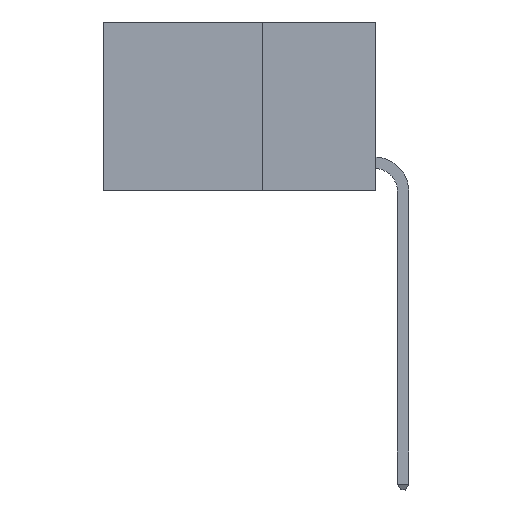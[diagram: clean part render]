
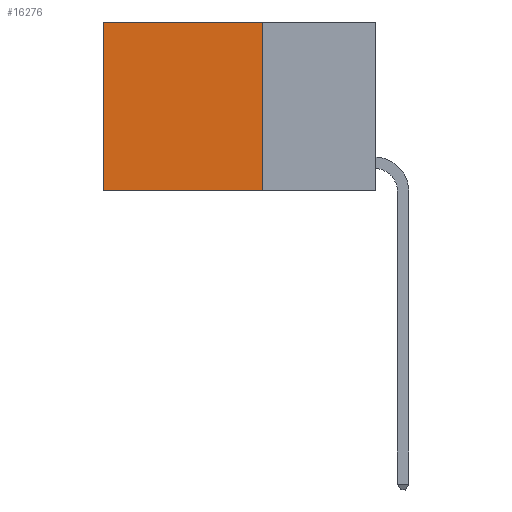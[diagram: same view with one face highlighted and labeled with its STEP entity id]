
A CAD part, left-side view. The second image highlights one B-rep face of the part: STEP entity #16276.
In plain terms, the highlighted planar face has unit normal (-1, 0, 0).
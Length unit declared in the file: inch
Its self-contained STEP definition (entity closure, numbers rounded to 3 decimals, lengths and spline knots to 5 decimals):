
#31 = CARTESIAN_POINT ( 'NONE',  ( 0.2625, 0.25, 0. ) ) ;
#176 = EDGE_CURVE ( 'NONE', #10624, #14972, #15602, .T. ) ;
#853 = LINE ( 'NONE', #31, #12790 ) ;
#1154 = CARTESIAN_POINT ( 'NONE',  ( 0.2625, 0.25, -0.37 ) ) ;
#1248 = DIRECTION ( 'NONE',  ( 0., 1., 0. ) ) ;
#1884 = DIRECTION ( 'NONE',  ( 0., 0., -1. ) ) ;
#3001 = VERTEX_POINT ( 'NONE', #10135 ) ;
#3259 = FACE_OUTER_BOUND ( 'NONE', #13086, .T. ) ;
#3706 = EDGE_CURVE ( 'NONE', #3001, #7408, #17821, .T. ) ;
#5511 = LINE ( 'NONE', #10163, #17362 ) ;
#6424 = CARTESIAN_POINT ( 'NONE',  ( 0.2625, 0.25, -0.37 ) ) ;
#7408 = VERTEX_POINT ( 'NONE', #14575 ) ;
#7544 = ORIENTED_EDGE ( 'NONE', *, *, #11592, .T. ) ;
#7986 = ORIENTED_EDGE ( 'NONE', *, *, #3706, .T. ) ;
#8156 = PLANE ( 'NONE',  #18578 ) ;
#9150 = VECTOR ( 'NONE', #14631, 39.37008 ) ;
#9650 = ORIENTED_EDGE ( 'NONE', *, *, #14235, .F. ) ;
#10135 = CARTESIAN_POINT ( 'NONE',  ( 0.2625, 0.25, 0. ) ) ;
#10163 = CARTESIAN_POINT ( 'NONE',  ( 0.2625, 0.6, 0. ) ) ;
#10624 = VERTEX_POINT ( 'NONE', #6424 ) ;
#11190 = DIRECTION ( 'NONE',  ( 1., 0., 0. ) ) ;
#11592 = EDGE_CURVE ( 'NONE', #7408, #14972, #5511, .T. ) ;
#12505 = DIRECTION ( 'NONE',  ( 0., 0., -1. ) ) ;
#12790 = VECTOR ( 'NONE', #12505, 39.37008 ) ;
#13086 = EDGE_LOOP ( 'NONE', ( #7544, #13265, #9650, #7986 ) ) ;
#13265 = ORIENTED_EDGE ( 'NONE', *, *, #176, .F. ) ;
#13368 = DIRECTION ( 'NONE',  ( 0., 0., -1. ) ) ;
#14235 = EDGE_CURVE ( 'NONE', #3001, #10624, #853, .T. ) ;
#14463 = CARTESIAN_POINT ( 'NONE',  ( 0.2625, 0.6, -0.37 ) ) ;
#14575 = CARTESIAN_POINT ( 'NONE',  ( 0.2625, 0.6, 0. ) ) ;
#14631 = DIRECTION ( 'NONE',  ( 0., 1., 0. ) ) ;
#14972 = VERTEX_POINT ( 'NONE', #14463 ) ;
#15602 = LINE ( 'NONE', #1154, #19606 ) ;
#15776 = CARTESIAN_POINT ( 'NONE',  ( 0.2625, 0.25, 0. ) ) ;
#16189 = CARTESIAN_POINT ( 'NONE',  ( 0.2625, 0.25, 0. ) ) ;
#16276 = ADVANCED_FACE ( 'NONE', ( #3259 ), #8156, .F. ) ;
#17362 = VECTOR ( 'NONE', #13368, 39.37008 ) ;
#17821 = LINE ( 'NONE', #16189, #9150 ) ;
#18578 = AXIS2_PLACEMENT_3D ( 'NONE', #15776, #11190, #1884 ) ;
#19606 = VECTOR ( 'NONE', #1248, 39.37008 ) ;
